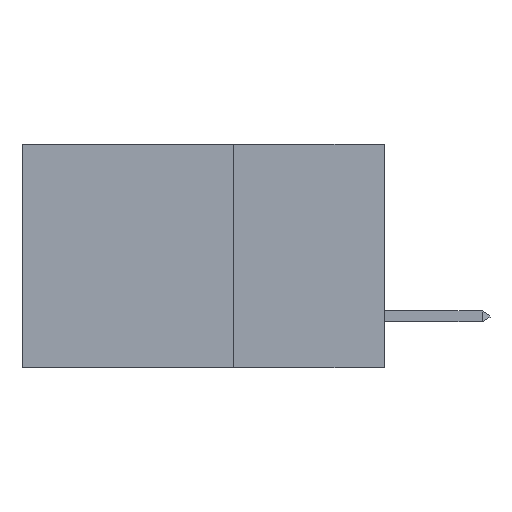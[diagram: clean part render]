
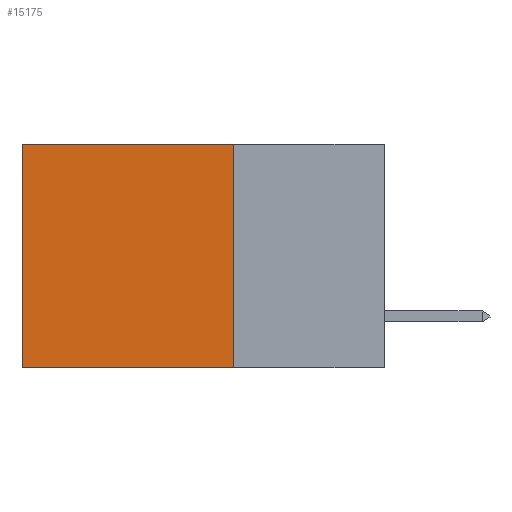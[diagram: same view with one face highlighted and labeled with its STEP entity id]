
A CAD part, left-side view. The second image highlights one B-rep face of the part: STEP entity #15175.
In plain terms, the highlighted planar face has unit normal (-1, 0, 0).
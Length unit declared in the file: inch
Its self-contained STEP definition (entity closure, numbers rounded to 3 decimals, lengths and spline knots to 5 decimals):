
#414 = DIRECTION ( 'NONE',  ( 0., 1., 0. ) ) ;
#871 = AXIS2_PLACEMENT_3D ( 'NONE', #12975, #34545, #16066 ) ;
#2545 = LINE ( 'NONE', #37743, #17851 ) ;
#3174 = ORIENTED_EDGE ( 'NONE', *, *, #15625, .T. ) ;
#6269 = CARTESIAN_POINT ( 'NONE',  ( 0.2875, 0.6, -0.37 ) ) ;
#6710 = LINE ( 'NONE', #21904, #21162 ) ;
#6975 = EDGE_LOOP ( 'NONE', ( #22629, #35664, #21838, #3174 ) ) ;
#8825 = LINE ( 'NONE', #33321, #24273 ) ;
#9721 = EDGE_CURVE ( 'NONE', #15697, #26672, #8825, .T. ) ;
#12975 = CARTESIAN_POINT ( 'NONE',  ( 0.2875, 0.25, 0. ) ) ;
#13254 = DIRECTION ( 'NONE',  ( 0., 0., -1. ) ) ;
#14042 = CARTESIAN_POINT ( 'NONE',  ( 0.2875, 0.25, -0.37 ) ) ;
#15175 = ADVANCED_FACE ( 'NONE', ( #37498 ), #28329, .F. ) ;
#15277 = VERTEX_POINT ( 'NONE', #22597 ) ;
#15625 = EDGE_CURVE ( 'NONE', #15697, #15277, #6710, .T. ) ;
#15697 = VERTEX_POINT ( 'NONE', #25232 ) ;
#16066 = DIRECTION ( 'NONE',  ( 0., 0., -1. ) ) ;
#17134 = DIRECTION ( 'NONE',  ( 0., 1., 0. ) ) ;
#17200 = EDGE_CURVE ( 'NONE', #26672, #27634, #19136, .T. ) ;
#17851 = VECTOR ( 'NONE', #13254, 39.37008 ) ;
#19136 = LINE ( 'NONE', #14042, #34568 ) ;
#21162 = VECTOR ( 'NONE', #414, 39.37008 ) ;
#21838 = ORIENTED_EDGE ( 'NONE', *, *, #9721, .F. ) ;
#21904 = CARTESIAN_POINT ( 'NONE',  ( 0.2875, 0.25, 0. ) ) ;
#22597 = CARTESIAN_POINT ( 'NONE',  ( 0.2875, 0.6, 0. ) ) ;
#22629 = ORIENTED_EDGE ( 'NONE', *, *, #29138, .T. ) ;
#24273 = VECTOR ( 'NONE', #36371, 39.37008 ) ;
#25232 = CARTESIAN_POINT ( 'NONE',  ( 0.2875, 0.25, 0. ) ) ;
#26435 = CARTESIAN_POINT ( 'NONE',  ( 0.2875, 0.25, -0.37 ) ) ;
#26672 = VERTEX_POINT ( 'NONE', #26435 ) ;
#27634 = VERTEX_POINT ( 'NONE', #6269 ) ;
#28329 = PLANE ( 'NONE',  #871 ) ;
#29138 = EDGE_CURVE ( 'NONE', #15277, #27634, #2545, .T. ) ;
#33321 = CARTESIAN_POINT ( 'NONE',  ( 0.2875, 0.25, 0. ) ) ;
#34545 = DIRECTION ( 'NONE',  ( 1., 0., 0. ) ) ;
#34568 = VECTOR ( 'NONE', #17134, 39.37008 ) ;
#35664 = ORIENTED_EDGE ( 'NONE', *, *, #17200, .F. ) ;
#36371 = DIRECTION ( 'NONE',  ( 0., 0., -1. ) ) ;
#37498 = FACE_OUTER_BOUND ( 'NONE', #6975, .T. ) ;
#37743 = CARTESIAN_POINT ( 'NONE',  ( 0.2875, 0.6, 0. ) ) ;
